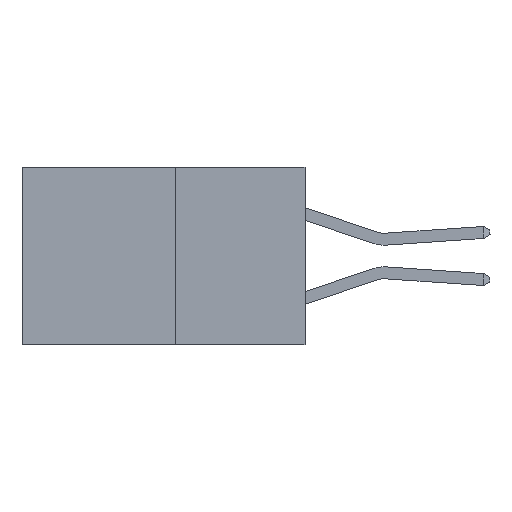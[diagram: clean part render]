
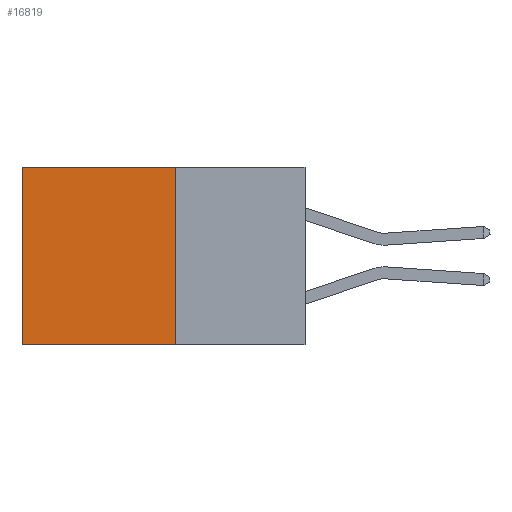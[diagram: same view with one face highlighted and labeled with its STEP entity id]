
A CAD part, left-side view. The second image highlights one B-rep face of the part: STEP entity #16819.
In plain terms, the highlighted planar face has unit normal (-1, 0, 0).
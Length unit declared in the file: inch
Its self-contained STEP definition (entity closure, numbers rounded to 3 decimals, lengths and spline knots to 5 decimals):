
#402 = VECTOR ( 'NONE', #10238, 39.37008 ) ;
#906 = DIRECTION ( 'NONE',  ( 0., 0., -1. ) ) ;
#1176 = EDGE_CURVE ( 'NONE', #15933, #8727, #9194, .T. ) ;
#2125 = EDGE_LOOP ( 'NONE', ( #4628, #8043, #10965, #4472 ) ) ;
#2198 = VECTOR ( 'NONE', #12865, 39.37008 ) ;
#3533 = LINE ( 'NONE', #11092, #7938 ) ;
#4472 = ORIENTED_EDGE ( 'NONE', *, *, #1176, .T. ) ;
#4600 = VERTEX_POINT ( 'NONE', #12578 ) ;
#4628 = ORIENTED_EDGE ( 'NONE', *, *, #6411, .T. ) ;
#4882 = DIRECTION ( 'NONE',  ( 0., 0., -1. ) ) ;
#4965 = CARTESIAN_POINT ( 'NONE',  ( 0.277, 0.59, -0.37 ) ) ;
#6411 = EDGE_CURVE ( 'NONE', #8727, #12586, #17284, .T. ) ;
#7396 = EDGE_CURVE ( 'NONE', #15933, #4600, #11487, .T. ) ;
#7572 = CARTESIAN_POINT ( 'NONE',  ( 0.277, 0.27, 0. ) ) ;
#7912 = CARTESIAN_POINT ( 'NONE',  ( 0.277, 0.27, -0.37 ) ) ;
#7938 = VECTOR ( 'NONE', #17493, 39.37008 ) ;
#8043 = ORIENTED_EDGE ( 'NONE', *, *, #10199, .F. ) ;
#8322 = CARTESIAN_POINT ( 'NONE',  ( 0.277, 0.59, -0.37 ) ) ;
#8727 = VERTEX_POINT ( 'NONE', #18909 ) ;
#9194 = LINE ( 'NONE', #7572, #402 ) ;
#10199 = EDGE_CURVE ( 'NONE', #4600, #12586, #3533, .T. ) ;
#10238 = DIRECTION ( 'NONE',  ( 0., 1., 0. ) ) ;
#10781 = DIRECTION ( 'NONE',  ( 1., 0., 0. ) ) ;
#10965 = ORIENTED_EDGE ( 'NONE', *, *, #7396, .F. ) ;
#11092 = CARTESIAN_POINT ( 'NONE',  ( 0.277, 0.27, -0.37 ) ) ;
#11126 = CARTESIAN_POINT ( 'NONE',  ( 0.277, 0.27, 0. ) ) ;
#11487 = LINE ( 'NONE', #7912, #2198 ) ;
#12578 = CARTESIAN_POINT ( 'NONE',  ( 0.277, 0.27, -0.37 ) ) ;
#12586 = VERTEX_POINT ( 'NONE', #8322 ) ;
#12865 = DIRECTION ( 'NONE',  ( 0., 0., -1. ) ) ;
#14703 = AXIS2_PLACEMENT_3D ( 'NONE', #15612, #10781, #906 ) ;
#15612 = CARTESIAN_POINT ( 'NONE',  ( 0.277, 0.27, -0.37 ) ) ;
#15933 = VERTEX_POINT ( 'NONE', #11126 ) ;
#16482 = FACE_OUTER_BOUND ( 'NONE', #2125, .T. ) ;
#16819 = ADVANCED_FACE ( 'NONE', ( #16482 ), #20334, .F. ) ;
#17284 = LINE ( 'NONE', #4965, #20467 ) ;
#17493 = DIRECTION ( 'NONE',  ( 0., 1., 0. ) ) ;
#18909 = CARTESIAN_POINT ( 'NONE',  ( 0.277, 0.59, 0. ) ) ;
#20334 = PLANE ( 'NONE',  #14703 ) ;
#20467 = VECTOR ( 'NONE', #4882, 39.37008 ) ;
